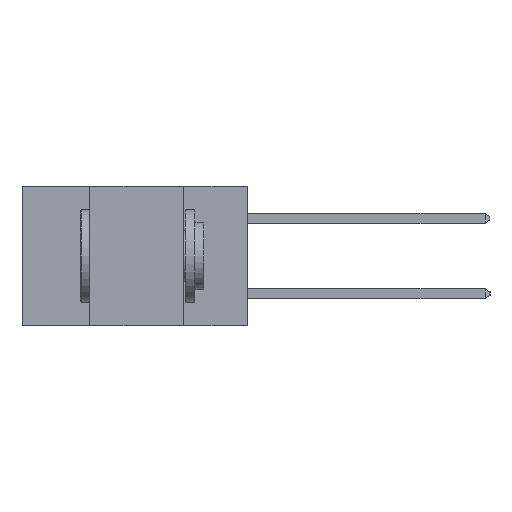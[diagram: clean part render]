
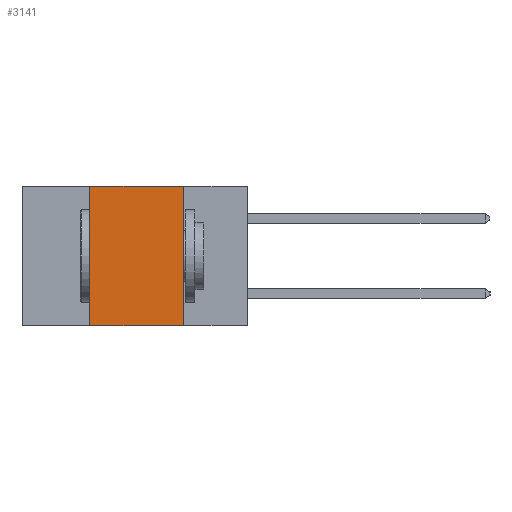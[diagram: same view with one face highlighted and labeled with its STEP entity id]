
A CAD part, left-side view. The second image highlights one B-rep face of the part: STEP entity #3141.
In plain terms, the highlighted planar face has unit normal (-1, 0, 0).
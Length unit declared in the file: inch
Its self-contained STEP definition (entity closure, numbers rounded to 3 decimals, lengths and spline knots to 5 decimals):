
#608 = CARTESIAN_POINT ( 'NONE',  ( 0., 0.6, -0.37 ) ) ;
#994 = CARTESIAN_POINT ( 'NONE',  ( 0., 0.6, 0. ) ) ;
#1435 = DIRECTION ( 'NONE',  ( 1., 0., 0. ) ) ;
#2399 = EDGE_CURVE ( 'NONE', #13017, #10101, #9281, .T. ) ;
#2549 = VERTEX_POINT ( 'NONE', #5895 ) ;
#2600 = LINE ( 'NONE', #15286, #5556 ) ;
#3141 = ADVANCED_FACE ( 'NONE', ( #3346 ), #10627, .F. ) ;
#3346 = FACE_OUTER_BOUND ( 'NONE', #6108, .T. ) ;
#3686 = CARTESIAN_POINT ( 'NONE',  ( 0., 0.17, 0. ) ) ;
#4010 = AXIS2_PLACEMENT_3D ( 'NONE', #10776, #1435, #8560 ) ;
#4099 = ORIENTED_EDGE ( 'NONE', *, *, #2399, .F. ) ;
#5556 = VECTOR ( 'NONE', #6713, 39.37008 ) ;
#5895 = CARTESIAN_POINT ( 'NONE',  ( 0., 0.17, -0.37 ) ) ;
#5987 = CARTESIAN_POINT ( 'NONE',  ( 0., 0.42, 0. ) ) ;
#6108 = EDGE_LOOP ( 'NONE', ( #15035, #4099, #12794, #12400 ) ) ;
#6398 = VECTOR ( 'NONE', #11473, 39.37008 ) ;
#6713 = DIRECTION ( 'NONE',  ( 0., 0., -1. ) ) ;
#7523 = VERTEX_POINT ( 'NONE', #11058 ) ;
#7734 = LINE ( 'NONE', #608, #13887 ) ;
#8560 = DIRECTION ( 'NONE',  ( 0., 0., -1. ) ) ;
#9281 = LINE ( 'NONE', #994, #9960 ) ;
#9642 = EDGE_CURVE ( 'NONE', #7523, #13017, #10078, .T. ) ;
#9960 = VECTOR ( 'NONE', #15402, 39.37008 ) ;
#10078 = LINE ( 'NONE', #10236, #6398 ) ;
#10101 = VERTEX_POINT ( 'NONE', #3686 ) ;
#10236 = CARTESIAN_POINT ( 'NONE',  ( 0., 0.42, -0.37 ) ) ;
#10627 = PLANE ( 'NONE',  #4010 ) ;
#10762 = EDGE_CURVE ( 'NONE', #7523, #2549, #7734, .T. ) ;
#10776 = CARTESIAN_POINT ( 'NONE',  ( 0., 0.6, 0. ) ) ;
#11058 = CARTESIAN_POINT ( 'NONE',  ( 0., 0.42, -0.37 ) ) ;
#11473 = DIRECTION ( 'NONE',  ( 0., 0., 1. ) ) ;
#12400 = ORIENTED_EDGE ( 'NONE', *, *, #10762, .T. ) ;
#12720 = EDGE_CURVE ( 'NONE', #10101, #2549, #2600, .T. ) ;
#12794 = ORIENTED_EDGE ( 'NONE', *, *, #9642, .F. ) ;
#13017 = VERTEX_POINT ( 'NONE', #5987 ) ;
#13887 = VECTOR ( 'NONE', #14232, 39.37008 ) ;
#14232 = DIRECTION ( 'NONE',  ( 0., -1., 0. ) ) ;
#15035 = ORIENTED_EDGE ( 'NONE', *, *, #12720, .F. ) ;
#15286 = CARTESIAN_POINT ( 'NONE',  ( 0., 0.17, -0.37 ) ) ;
#15402 = DIRECTION ( 'NONE',  ( 0., -1., 0. ) ) ;
